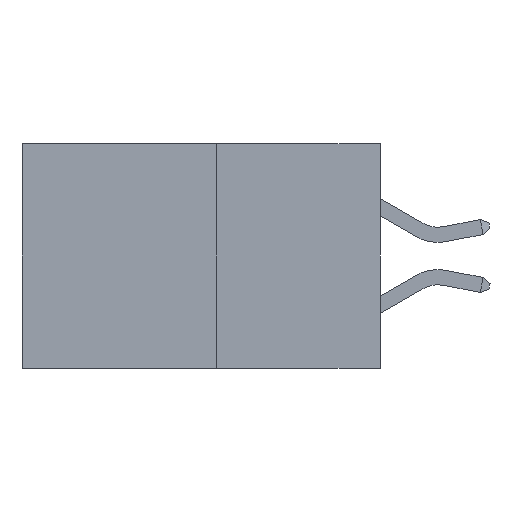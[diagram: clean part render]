
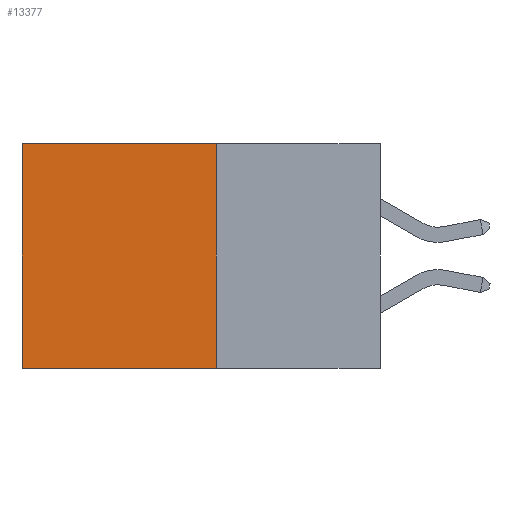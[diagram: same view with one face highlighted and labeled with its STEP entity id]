
A CAD part, left-side view. The second image highlights one B-rep face of the part: STEP entity #13377.
In plain terms, the highlighted planar face has unit normal (-1, 0, 0).
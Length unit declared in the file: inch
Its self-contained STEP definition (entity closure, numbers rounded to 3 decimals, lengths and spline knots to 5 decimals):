
#982 = EDGE_CURVE ( 'NONE', #11528, #4562, #6552, .T. ) ;
#1279 = VECTOR ( 'NONE', #8548, 39.37008 ) ;
#1703 = VECTOR ( 'NONE', #2318, 39.37008 ) ;
#2063 = PLANE ( 'NONE',  #2312 ) ;
#2312 = AXIS2_PLACEMENT_3D ( 'NONE', #8240, #3334, #11920 ) ;
#2318 = DIRECTION ( 'NONE',  ( 0., 0., -1. ) ) ;
#2625 = LINE ( 'NONE', #15104, #3558 ) ;
#3334 = DIRECTION ( 'NONE',  ( 1., 0., 0. ) ) ;
#3558 = VECTOR ( 'NONE', #6675, 39.37008 ) ;
#3645 = EDGE_CURVE ( 'NONE', #7367, #4562, #11470, .T. ) ;
#4562 = VERTEX_POINT ( 'NONE', #10197 ) ;
#4590 = EDGE_CURVE ( 'NONE', #7647, #11528, #7478, .T. ) ;
#4992 = CARTESIAN_POINT ( 'NONE',  ( 0.277, 0.27, 0. ) ) ;
#6301 = DIRECTION ( 'NONE',  ( 0., 1., 0. ) ) ;
#6538 = CARTESIAN_POINT ( 'NONE',  ( 0.277, 0.27, -0.37 ) ) ;
#6552 = LINE ( 'NONE', #6538, #13330 ) ;
#6675 = DIRECTION ( 'NONE',  ( 0., 1., 0. ) ) ;
#6803 = CARTESIAN_POINT ( 'NONE',  ( 0.277, 0.27, -0.37 ) ) ;
#7367 = VERTEX_POINT ( 'NONE', #8769 ) ;
#7478 = LINE ( 'NONE', #8537, #1279 ) ;
#7647 = VERTEX_POINT ( 'NONE', #4992 ) ;
#7970 = ORIENTED_EDGE ( 'NONE', *, *, #3645, .T. ) ;
#8240 = CARTESIAN_POINT ( 'NONE',  ( 0.277, 0.27, -0.37 ) ) ;
#8537 = CARTESIAN_POINT ( 'NONE',  ( 0.277, 0.27, -0.37 ) ) ;
#8548 = DIRECTION ( 'NONE',  ( 0., 0., -1. ) ) ;
#8769 = CARTESIAN_POINT ( 'NONE',  ( 0.277, 0.59, 0. ) ) ;
#8886 = ORIENTED_EDGE ( 'NONE', *, *, #982, .F. ) ;
#9575 = FACE_OUTER_BOUND ( 'NONE', #13015, .T. ) ;
#10180 = EDGE_CURVE ( 'NONE', #7647, #7367, #2625, .T. ) ;
#10197 = CARTESIAN_POINT ( 'NONE',  ( 0.277, 0.59, -0.37 ) ) ;
#11328 = ORIENTED_EDGE ( 'NONE', *, *, #4590, .F. ) ;
#11470 = LINE ( 'NONE', #13883, #1703 ) ;
#11528 = VERTEX_POINT ( 'NONE', #6803 ) ;
#11920 = DIRECTION ( 'NONE',  ( 0., 0., -1. ) ) ;
#13015 = EDGE_LOOP ( 'NONE', ( #7970, #8886, #11328, #15105 ) ) ;
#13330 = VECTOR ( 'NONE', #6301, 39.37008 ) ;
#13377 = ADVANCED_FACE ( 'NONE', ( #9575 ), #2063, .F. ) ;
#13883 = CARTESIAN_POINT ( 'NONE',  ( 0.277, 0.59, -0.37 ) ) ;
#15104 = CARTESIAN_POINT ( 'NONE',  ( 0.277, 0.27, 0. ) ) ;
#15105 = ORIENTED_EDGE ( 'NONE', *, *, #10180, .T. ) ;
